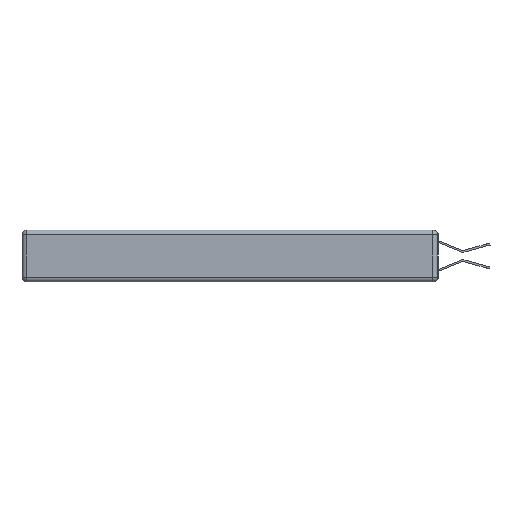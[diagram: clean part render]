
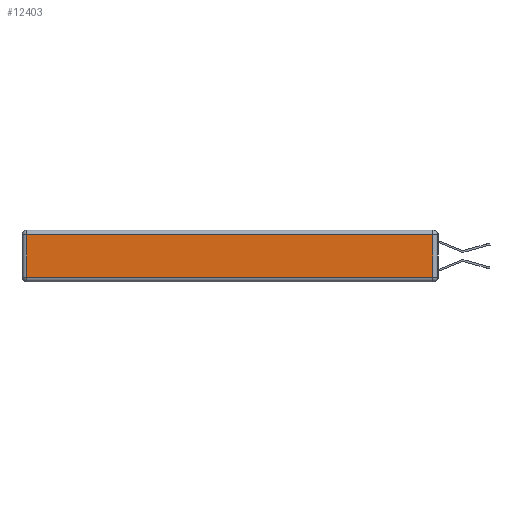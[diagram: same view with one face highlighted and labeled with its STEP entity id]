
A CAD part, left-side view. The second image highlights one B-rep face of the part: STEP entity #12403.
In plain terms, the highlighted planar face has unit normal (-1, 0, 0).
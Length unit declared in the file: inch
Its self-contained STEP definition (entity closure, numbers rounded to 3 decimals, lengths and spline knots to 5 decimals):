
#250 = VERTEX_POINT ( 'NONE', #12011 ) ;
#374 = ORIENTED_EDGE ( 'NONE', *, *, #422, .T. ) ;
#396 = VECTOR ( 'NONE', #11608, 39.37008 ) ;
#422 = EDGE_CURVE ( 'NONE', #9817, #2814, #3347, .T. ) ;
#804 = DIRECTION ( 'NONE',  ( 0., 0., -1. ) ) ;
#1350 = DIRECTION ( 'NONE',  ( 0., 1., 0. ) ) ;
#1760 = DIRECTION ( 'NONE',  ( 0., 0., 1. ) ) ;
#2128 = EDGE_CURVE ( 'NONE', #250, #8701, #8345, .T. ) ;
#2814 = VERTEX_POINT ( 'NONE', #5523 ) ;
#2836 = CARTESIAN_POINT ( 'NONE',  ( 0., 2.72, -0.343 ) ) ;
#3347 = LINE ( 'NONE', #2836, #12006 ) ;
#3850 = CARTESIAN_POINT ( 'NONE',  ( 0., 0., -0.343 ) ) ;
#4357 = CARTESIAN_POINT ( 'NONE',  ( 0., 2.72, -0.03 ) ) ;
#4463 = EDGE_LOOP ( 'NONE', ( #11175, #7552, #5895, #374 ) ) ;
#4788 = DIRECTION ( 'NONE',  ( -1., 0., 0. ) ) ;
#5452 = EDGE_CURVE ( 'NONE', #8701, #9817, #9680, .T. ) ;
#5523 = CARTESIAN_POINT ( 'NONE',  ( 0., 2.72, -0.313 ) ) ;
#5678 = VECTOR ( 'NONE', #11948, 39.37008 ) ;
#5693 = CARTESIAN_POINT ( 'NONE',  ( 0., 0.03, -0.343 ) ) ;
#5895 = ORIENTED_EDGE ( 'NONE', *, *, #5452, .T. ) ;
#6254 = CARTESIAN_POINT ( 'NONE',  ( 0., 0.03, -0.03 ) ) ;
#6487 = EDGE_CURVE ( 'NONE', #2814, #250, #8256, .T. ) ;
#7523 = AXIS2_PLACEMENT_3D ( 'NONE', #3850, #4788, #1760 ) ;
#7552 = ORIENTED_EDGE ( 'NONE', *, *, #2128, .T. ) ;
#8138 = VECTOR ( 'NONE', #1350, 39.37008 ) ;
#8256 = LINE ( 'NONE', #9019, #5678 ) ;
#8345 = LINE ( 'NONE', #5693, #396 ) ;
#8701 = VERTEX_POINT ( 'NONE', #6254 ) ;
#8776 = PLANE ( 'NONE',  #7523 ) ;
#9019 = CARTESIAN_POINT ( 'NONE',  ( 0., 0., -0.313 ) ) ;
#9680 = LINE ( 'NONE', #10202, #8138 ) ;
#9817 = VERTEX_POINT ( 'NONE', #4357 ) ;
#10202 = CARTESIAN_POINT ( 'NONE',  ( 0., 2.75, -0.03 ) ) ;
#10700 = FACE_OUTER_BOUND ( 'NONE', #4463, .T. ) ;
#11175 = ORIENTED_EDGE ( 'NONE', *, *, #6487, .T. ) ;
#11608 = DIRECTION ( 'NONE',  ( 0., 0., 1. ) ) ;
#11948 = DIRECTION ( 'NONE',  ( 0., -1., 0. ) ) ;
#12006 = VECTOR ( 'NONE', #804, 39.37008 ) ;
#12011 = CARTESIAN_POINT ( 'NONE',  ( 0., 0.03, -0.313 ) ) ;
#12403 = ADVANCED_FACE ( 'NONE', ( #10700 ), #8776, .T. ) ;
